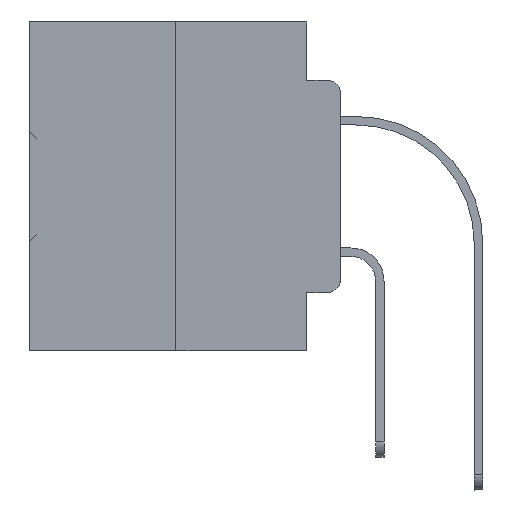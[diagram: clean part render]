
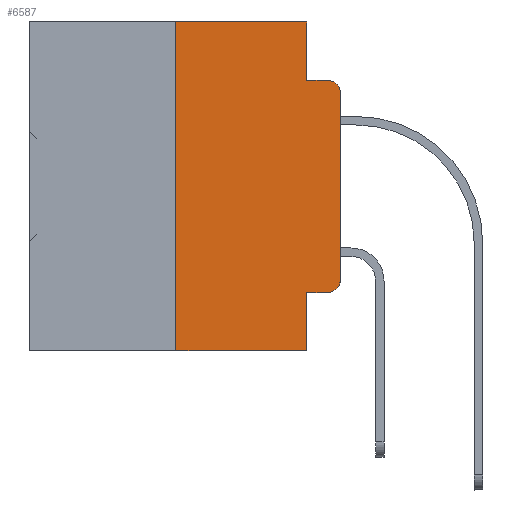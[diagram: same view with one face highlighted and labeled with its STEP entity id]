
A CAD part, left-side view. The second image highlights one B-rep face of the part: STEP entity #6587.
In plain terms, the highlighted planar face has unit normal (-1, 0, 0).
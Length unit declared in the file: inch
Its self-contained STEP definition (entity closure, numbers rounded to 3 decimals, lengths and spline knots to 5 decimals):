
#755 = CARTESIAN_POINT ( 'NONE',  ( 0., 0.02, -0.4115 ) ) ;
#1506 = DIRECTION ( 'NONE',  ( 0., 0., 1. ) ) ;
#2296 = EDGE_CURVE ( 'NONE', #23987, #7453, #13872, .T. ) ;
#3174 = VECTOR ( 'NONE', #31684, 39.37008 ) ;
#3498 = VERTEX_POINT ( 'NONE', #18847 ) ;
#4438 = EDGE_CURVE ( 'NONE', #7453, #18356, #23902, .T. ) ;
#4451 = CARTESIAN_POINT ( 'NONE',  ( 0., 0., -0.1085 ) ) ;
#4481 = LINE ( 'NONE', #8167, #35781 ) ;
#4521 = DIRECTION ( 'NONE',  ( 0., 0., -1. ) ) ;
#5005 = EDGE_CURVE ( 'NONE', #17015, #13108, #18227, .T. ) ;
#5541 = LINE ( 'NONE', #36979, #15884 ) ;
#6587 = ADVANCED_FACE ( 'NONE', ( #19640 ), #17390, .F. ) ;
#6596 = CARTESIAN_POINT ( 'NONE',  ( 0., 0.051, -0.0885 ) ) ;
#6795 = CARTESIAN_POINT ( 'NONE',  ( 0., 0.25, 0. ) ) ;
#7150 = VERTEX_POINT ( 'NONE', #23879 ) ;
#7453 = VERTEX_POINT ( 'NONE', #755 ) ;
#8160 = CARTESIAN_POINT ( 'NONE',  ( 0., 0.02, -0.0885 ) ) ;
#8167 = CARTESIAN_POINT ( 'NONE',  ( 0., 0.051, 0. ) ) ;
#8242 = CARTESIAN_POINT ( 'NONE',  ( 0., 0.25, 0. ) ) ;
#8387 = VECTOR ( 'NONE', #38791, 39.37008 ) ;
#8481 = CARTESIAN_POINT ( 'NONE',  ( 0., 0.02, -0.3915 ) ) ;
#9522 = CARTESIAN_POINT ( 'NONE',  ( 0., 0.473, -0.5 ) ) ;
#10937 = EDGE_LOOP ( 'NONE', ( #22093, #32977, #20770, #32638, #20922, #39721, #37399, #15850, #22925, #18613 ) ) ;
#11502 = AXIS2_PLACEMENT_3D ( 'NONE', #8481, #11550, #27257 ) ;
#11550 = DIRECTION ( 'NONE',  ( -1., 0., 0. ) ) ;
#12353 = EDGE_CURVE ( 'NONE', #3498, #17015, #29479, .T. ) ;
#12593 = EDGE_CURVE ( 'NONE', #7150, #14548, #25173, .T. ) ;
#13108 = VERTEX_POINT ( 'NONE', #21660 ) ;
#13337 = VECTOR ( 'NONE', #23878, 39.37008 ) ;
#13509 = CARTESIAN_POINT ( 'NONE',  ( 0., 0.473, 0. ) ) ;
#13872 = LINE ( 'NONE', #20796, #8387 ) ;
#14241 = EDGE_CURVE ( 'NONE', #13108, #7150, #5541, .T. ) ;
#14548 = VERTEX_POINT ( 'NONE', #8160 ) ;
#15338 = DIRECTION ( 'NONE',  ( 0., 0., -1. ) ) ;
#15451 = DIRECTION ( 'NONE',  ( 0., -1., 0. ) ) ;
#15466 = VECTOR ( 'NONE', #17832, 39.37008 ) ;
#15792 = CARTESIAN_POINT ( 'NONE',  ( 0., 0., -0.3915 ) ) ;
#15850 = ORIENTED_EDGE ( 'NONE', *, *, #15883, .F. ) ;
#15883 = EDGE_CURVE ( 'NONE', #23987, #18062, #4481, .T. ) ;
#15884 = VECTOR ( 'NONE', #15338, 39.37008 ) ;
#17015 = VERTEX_POINT ( 'NONE', #6795 ) ;
#17222 = VECTOR ( 'NONE', #15451, 39.37008 ) ;
#17390 = PLANE ( 'NONE',  #33191 ) ;
#17832 = DIRECTION ( 'NONE',  ( 0., -1., 0. ) ) ;
#18062 = VERTEX_POINT ( 'NONE', #19158 ) ;
#18227 = LINE ( 'NONE', #21289, #15466 ) ;
#18356 = VERTEX_POINT ( 'NONE', #15792 ) ;
#18613 = ORIENTED_EDGE ( 'NONE', *, *, #4438, .T. ) ;
#18847 = CARTESIAN_POINT ( 'NONE',  ( 0., 0.25, -0.5 ) ) ;
#19158 = CARTESIAN_POINT ( 'NONE',  ( 0., 0.051, -0.5 ) ) ;
#19640 = FACE_OUTER_BOUND ( 'NONE', #10937, .T. ) ;
#20770 = ORIENTED_EDGE ( 'NONE', *, *, #12593, .F. ) ;
#20796 = CARTESIAN_POINT ( 'NONE',  ( 0., 0.051, -0.4115 ) ) ;
#20922 = ORIENTED_EDGE ( 'NONE', *, *, #5005, .F. ) ;
#21289 = CARTESIAN_POINT ( 'NONE',  ( 0., 0.473, 0. ) ) ;
#21582 = LINE ( 'NONE', #9522, #17222 ) ;
#21660 = CARTESIAN_POINT ( 'NONE',  ( 0., 0.051, 0. ) ) ;
#22093 = ORIENTED_EDGE ( 'NONE', *, *, #25064, .T. ) ;
#22658 = EDGE_CURVE ( 'NONE', #3498, #18062, #21582, .T. ) ;
#22925 = ORIENTED_EDGE ( 'NONE', *, *, #2296, .T. ) ;
#23878 = DIRECTION ( 'NONE',  ( 0., 0., 1. ) ) ;
#23879 = CARTESIAN_POINT ( 'NONE',  ( 0., 0.051, -0.0885 ) ) ;
#23902 = CIRCLE ( 'NONE', #11502, 0.02 ) ;
#23987 = VERTEX_POINT ( 'NONE', #37719 ) ;
#24462 = AXIS2_PLACEMENT_3D ( 'NONE', #29709, #36661, #32983 ) ;
#25064 = EDGE_CURVE ( 'NONE', #18356, #30867, #37434, .T. ) ;
#25173 = LINE ( 'NONE', #6596, #3174 ) ;
#26570 = DIRECTION ( 'NONE',  ( 1., 0., 0. ) ) ;
#27257 = DIRECTION ( 'NONE',  ( 0., 0., -1. ) ) ;
#29479 = LINE ( 'NONE', #8242, #39706 ) ;
#29493 = EDGE_CURVE ( 'NONE', #30867, #14548, #29665, .T. ) ;
#29665 = CIRCLE ( 'NONE', #24462, 0.02 ) ;
#29709 = CARTESIAN_POINT ( 'NONE',  ( 0., 0.02, -0.1085 ) ) ;
#30867 = VERTEX_POINT ( 'NONE', #4451 ) ;
#31684 = DIRECTION ( 'NONE',  ( 0., -1., 0. ) ) ;
#32638 = ORIENTED_EDGE ( 'NONE', *, *, #14241, .F. ) ;
#32878 = DIRECTION ( 'NONE',  ( 0., 0., -1. ) ) ;
#32977 = ORIENTED_EDGE ( 'NONE', *, *, #29493, .T. ) ;
#32983 = DIRECTION ( 'NONE',  ( 0., 0., -1. ) ) ;
#33191 = AXIS2_PLACEMENT_3D ( 'NONE', #13509, #26570, #4521 ) ;
#35781 = VECTOR ( 'NONE', #32878, 39.37008 ) ;
#36661 = DIRECTION ( 'NONE',  ( -1., 0., 0. ) ) ;
#36979 = CARTESIAN_POINT ( 'NONE',  ( 0., 0.051, 0. ) ) ;
#37399 = ORIENTED_EDGE ( 'NONE', *, *, #22658, .T. ) ;
#37434 = LINE ( 'NONE', #38181, #13337 ) ;
#37719 = CARTESIAN_POINT ( 'NONE',  ( 0., 0.051, -0.4115 ) ) ;
#38181 = CARTESIAN_POINT ( 'NONE',  ( 0., 0., 0. ) ) ;
#38791 = DIRECTION ( 'NONE',  ( 0., -1., 0. ) ) ;
#39706 = VECTOR ( 'NONE', #1506, 39.37008 ) ;
#39721 = ORIENTED_EDGE ( 'NONE', *, *, #12353, .F. ) ;
